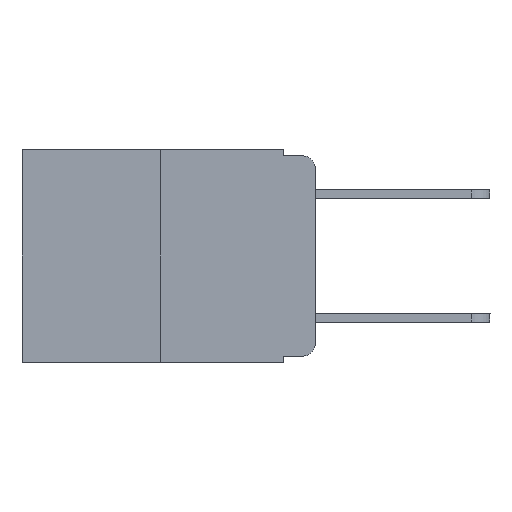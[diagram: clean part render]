
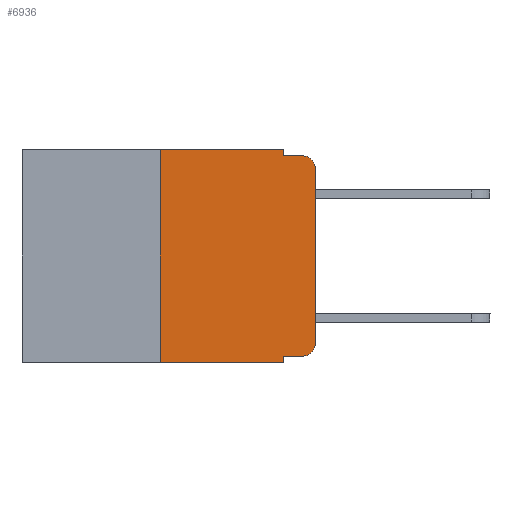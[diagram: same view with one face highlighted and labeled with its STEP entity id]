
A CAD part, left-side view. The second image highlights one B-rep face of the part: STEP entity #6936.
In plain terms, the highlighted planar face has unit normal (-1, 0, 0).
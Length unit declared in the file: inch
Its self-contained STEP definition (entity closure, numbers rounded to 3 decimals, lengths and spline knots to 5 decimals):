
#98 = VERTEX_POINT ( 'NONE', #1448 ) ;
#138 = CARTESIAN_POINT ( 'NONE',  ( 0., 0., -0.313 ) ) ;
#266 = ORIENTED_EDGE ( 'NONE', *, *, #9461, .T. ) ;
#419 = FACE_OUTER_BOUND ( 'NONE', #4440, .T. ) ;
#477 = VECTOR ( 'NONE', #10272, 39.37008 ) ;
#665 = CARTESIAN_POINT ( 'NONE',  ( 0., 0.25, 0. ) ) ;
#826 = DIRECTION ( 'NONE',  ( 0., -1., 0. ) ) ;
#852 = VERTEX_POINT ( 'NONE', #5636 ) ;
#1002 = CIRCLE ( 'NONE', #3385, 0.02 ) ;
#1005 = EDGE_CURVE ( 'NONE', #98, #1396, #2122, .T. ) ;
#1047 = VECTOR ( 'NONE', #7690, 39.37008 ) ;
#1117 = CARTESIAN_POINT ( 'NONE',  ( 0., 0.051, 0. ) ) ;
#1147 = DIRECTION ( 'NONE',  ( 0., 0., -1. ) ) ;
#1150 = LINE ( 'NONE', #3912, #11850 ) ;
#1242 = DIRECTION ( 'NONE',  ( -1., 0., 0. ) ) ;
#1396 = VERTEX_POINT ( 'NONE', #11403 ) ;
#1404 = LINE ( 'NONE', #665, #5906 ) ;
#1448 = CARTESIAN_POINT ( 'NONE',  ( 0., 0., -0.03 ) ) ;
#1638 = DIRECTION ( 'NONE',  ( 0., 0., 1. ) ) ;
#1853 = CARTESIAN_POINT ( 'NONE',  ( 0., 0.051, -0.343 ) ) ;
#2096 = LINE ( 'NONE', #11086, #1047 ) ;
#2122 = CIRCLE ( 'NONE', #5765, 0.02 ) ;
#2709 = CARTESIAN_POINT ( 'NONE',  ( 0., 0.25, 0. ) ) ;
#2785 = VECTOR ( 'NONE', #826, 39.37008 ) ;
#2984 = EDGE_CURVE ( 'NONE', #852, #10252, #8857, .T. ) ;
#2997 = ORIENTED_EDGE ( 'NONE', *, *, #11982, .F. ) ;
#3063 = VERTEX_POINT ( 'NONE', #138 ) ;
#3385 = AXIS2_PLACEMENT_3D ( 'NONE', #11760, #1242, #5071 ) ;
#3440 = EDGE_CURVE ( 'NONE', #3063, #98, #10345, .T. ) ;
#3659 = EDGE_CURVE ( 'NONE', #12156, #4798, #1150, .T. ) ;
#3661 = DIRECTION ( 'NONE',  ( 0., 0., 1. ) ) ;
#3912 = CARTESIAN_POINT ( 'NONE',  ( 0., 0.473, 0. ) ) ;
#4111 = ORIENTED_EDGE ( 'NONE', *, *, #8232, .F. ) ;
#4213 = CARTESIAN_POINT ( 'NONE',  ( 0., 0.051, -0.01 ) ) ;
#4440 = EDGE_LOOP ( 'NONE', ( #12060, #12472, #2997, #4111, #11515, #7333, #7854, #10133, #266, #10895 ) ) ;
#4547 = VERTEX_POINT ( 'NONE', #12151 ) ;
#4798 = VERTEX_POINT ( 'NONE', #1117 ) ;
#4903 = DIRECTION ( 'NONE',  ( 0., -1., 0. ) ) ;
#4982 = CARTESIAN_POINT ( 'NONE',  ( 0., 0.051, 0. ) ) ;
#4987 = CARTESIAN_POINT ( 'NONE',  ( 0., 0.473, -0.343 ) ) ;
#5071 = DIRECTION ( 'NONE',  ( 0., 0., -1. ) ) ;
#5317 = VERTEX_POINT ( 'NONE', #7603 ) ;
#5636 = CARTESIAN_POINT ( 'NONE',  ( 0., 0.25, -0.343 ) ) ;
#5665 = DIRECTION ( 'NONE',  ( 1., 0., 0. ) ) ;
#5765 = AXIS2_PLACEMENT_3D ( 'NONE', #8790, #6826, #7787 ) ;
#5906 = VECTOR ( 'NONE', #1638, 39.37008 ) ;
#5912 = EDGE_CURVE ( 'NONE', #852, #12156, #1404, .T. ) ;
#6826 = DIRECTION ( 'NONE',  ( -1., 0., 0. ) ) ;
#6875 = LINE ( 'NONE', #4213, #2785 ) ;
#6936 = ADVANCED_FACE ( 'NONE', ( #419 ), #10461, .F. ) ;
#7333 = ORIENTED_EDGE ( 'NONE', *, *, #5912, .F. ) ;
#7353 = VECTOR ( 'NONE', #4903, 39.37008 ) ;
#7502 = CARTESIAN_POINT ( 'NONE',  ( 0., 0.051, 0. ) ) ;
#7603 = CARTESIAN_POINT ( 'NONE',  ( 0., 0.051, -0.01 ) ) ;
#7690 = DIRECTION ( 'NONE',  ( 0., -1., 0. ) ) ;
#7787 = DIRECTION ( 'NONE',  ( 0., 0., -1. ) ) ;
#7854 = ORIENTED_EDGE ( 'NONE', *, *, #2984, .T. ) ;
#8232 = EDGE_CURVE ( 'NONE', #4798, #5317, #11768, .T. ) ;
#8288 = LINE ( 'NONE', #4982, #9190 ) ;
#8541 = VECTOR ( 'NONE', #3661, 39.37008 ) ;
#8753 = AXIS2_PLACEMENT_3D ( 'NONE', #11313, #5665, #9558 ) ;
#8790 = CARTESIAN_POINT ( 'NONE',  ( 0., 0.02, -0.03 ) ) ;
#8857 = LINE ( 'NONE', #4987, #7353 ) ;
#8927 = EDGE_CURVE ( 'NONE', #4547, #10252, #8288, .T. ) ;
#9190 = VECTOR ( 'NONE', #1147, 39.37008 ) ;
#9461 = EDGE_CURVE ( 'NONE', #4547, #10167, #2096, .T. ) ;
#9558 = DIRECTION ( 'NONE',  ( 0., 0., -1. ) ) ;
#10133 = ORIENTED_EDGE ( 'NONE', *, *, #8927, .F. ) ;
#10167 = VERTEX_POINT ( 'NONE', #12171 ) ;
#10252 = VERTEX_POINT ( 'NONE', #1853 ) ;
#10272 = DIRECTION ( 'NONE',  ( 0., 0., -1. ) ) ;
#10345 = LINE ( 'NONE', #11379, #8541 ) ;
#10461 = PLANE ( 'NONE',  #8753 ) ;
#10895 = ORIENTED_EDGE ( 'NONE', *, *, #11111, .T. ) ;
#11086 = CARTESIAN_POINT ( 'NONE',  ( 0., 0.051, -0.333 ) ) ;
#11111 = EDGE_CURVE ( 'NONE', #10167, #3063, #1002, .T. ) ;
#11313 = CARTESIAN_POINT ( 'NONE',  ( 0., 0.473, 0. ) ) ;
#11379 = CARTESIAN_POINT ( 'NONE',  ( 0., 0., 0. ) ) ;
#11403 = CARTESIAN_POINT ( 'NONE',  ( 0., 0.02, -0.01 ) ) ;
#11515 = ORIENTED_EDGE ( 'NONE', *, *, #3659, .F. ) ;
#11620 = DIRECTION ( 'NONE',  ( 0., -1., 0. ) ) ;
#11760 = CARTESIAN_POINT ( 'NONE',  ( 0., 0.02, -0.313 ) ) ;
#11768 = LINE ( 'NONE', #7502, #477 ) ;
#11850 = VECTOR ( 'NONE', #11620, 39.37008 ) ;
#11982 = EDGE_CURVE ( 'NONE', #5317, #1396, #6875, .T. ) ;
#12060 = ORIENTED_EDGE ( 'NONE', *, *, #3440, .T. ) ;
#12151 = CARTESIAN_POINT ( 'NONE',  ( 0., 0.051, -0.333 ) ) ;
#12156 = VERTEX_POINT ( 'NONE', #2709 ) ;
#12171 = CARTESIAN_POINT ( 'NONE',  ( 0., 0.02, -0.333 ) ) ;
#12472 = ORIENTED_EDGE ( 'NONE', *, *, #1005, .T. ) ;
